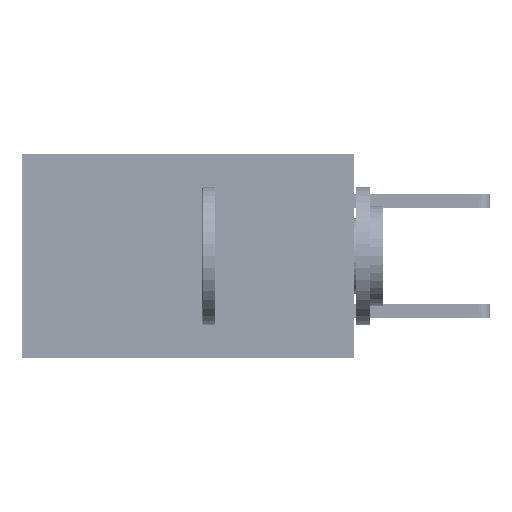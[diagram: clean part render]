
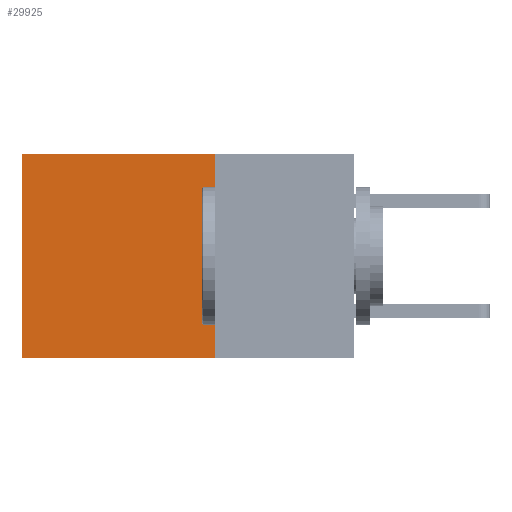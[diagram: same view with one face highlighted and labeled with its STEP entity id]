
A CAD part, left-side view. The second image highlights one B-rep face of the part: STEP entity #29925.
In plain terms, the highlighted planar face has unit normal (-1, 0, 0).
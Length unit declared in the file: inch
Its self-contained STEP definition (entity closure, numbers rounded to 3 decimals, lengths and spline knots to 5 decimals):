
#314 = CARTESIAN_POINT ( 'NONE',  ( 0.2875, 0.6, 0. ) ) ;
#1520 = PLANE ( 'NONE',  #20075 ) ;
#2114 = LINE ( 'NONE', #35898, #6044 ) ;
#5835 = DIRECTION ( 'NONE',  ( 0., 0., -1. ) ) ;
#6044 = VECTOR ( 'NONE', #5835, 39.37008 ) ;
#6503 = EDGE_CURVE ( 'NONE', #14254, #11322, #41241, .T. ) ;
#7307 = EDGE_LOOP ( 'NONE', ( #42453, #14765, #10799, #31300 ) ) ;
#10567 = EDGE_CURVE ( 'NONE', #11322, #31192, #21449, .T. ) ;
#10799 = ORIENTED_EDGE ( 'NONE', *, *, #19064, .F. ) ;
#11322 = VERTEX_POINT ( 'NONE', #314 ) ;
#12222 = CARTESIAN_POINT ( 'NONE',  ( 0.2875, 0.25, -0.37 ) ) ;
#12413 = VECTOR ( 'NONE', #21192, 39.37008 ) ;
#14254 = VERTEX_POINT ( 'NONE', #15453 ) ;
#14443 = CARTESIAN_POINT ( 'NONE',  ( 0.2875, 0.6, 0. ) ) ;
#14765 = ORIENTED_EDGE ( 'NONE', *, *, #35927, .F. ) ;
#14900 = DIRECTION ( 'NONE',  ( 0., 0., -1. ) ) ;
#15453 = CARTESIAN_POINT ( 'NONE',  ( 0.2875, 0.25, 0. ) ) ;
#18473 = VECTOR ( 'NONE', #34837, 39.37008 ) ;
#19064 = EDGE_CURVE ( 'NONE', #14254, #21073, #2114, .T. ) ;
#20075 = AXIS2_PLACEMENT_3D ( 'NONE', #24564, #41232, #14900 ) ;
#21073 = VERTEX_POINT ( 'NONE', #12222 ) ;
#21192 = DIRECTION ( 'NONE',  ( 0., 1., 0. ) ) ;
#21449 = LINE ( 'NONE', #14443, #18473 ) ;
#21831 = CARTESIAN_POINT ( 'NONE',  ( 0.2875, 0.25, -0.37 ) ) ;
#24564 = CARTESIAN_POINT ( 'NONE',  ( 0.2875, 0.25, 0. ) ) ;
#24686 = LINE ( 'NONE', #21831, #12413 ) ;
#24774 = FACE_OUTER_BOUND ( 'NONE', #7307, .T. ) ;
#29925 = ADVANCED_FACE ( 'NONE', ( #24774 ), #1520, .F. ) ;
#31192 = VERTEX_POINT ( 'NONE', #35095 ) ;
#31300 = ORIENTED_EDGE ( 'NONE', *, *, #6503, .T. ) ;
#34668 = CARTESIAN_POINT ( 'NONE',  ( 0.2875, 0.25, 0. ) ) ;
#34837 = DIRECTION ( 'NONE',  ( 0., 0., -1. ) ) ;
#35095 = CARTESIAN_POINT ( 'NONE',  ( 0.2875, 0.6, -0.37 ) ) ;
#35898 = CARTESIAN_POINT ( 'NONE',  ( 0.2875, 0.25, 0. ) ) ;
#35927 = EDGE_CURVE ( 'NONE', #21073, #31192, #24686, .T. ) ;
#40122 = VECTOR ( 'NONE', #41454, 39.37008 ) ;
#41232 = DIRECTION ( 'NONE',  ( 1., 0., 0. ) ) ;
#41241 = LINE ( 'NONE', #34668, #40122 ) ;
#41454 = DIRECTION ( 'NONE',  ( 0., 1., 0. ) ) ;
#42453 = ORIENTED_EDGE ( 'NONE', *, *, #10567, .T. ) ;
